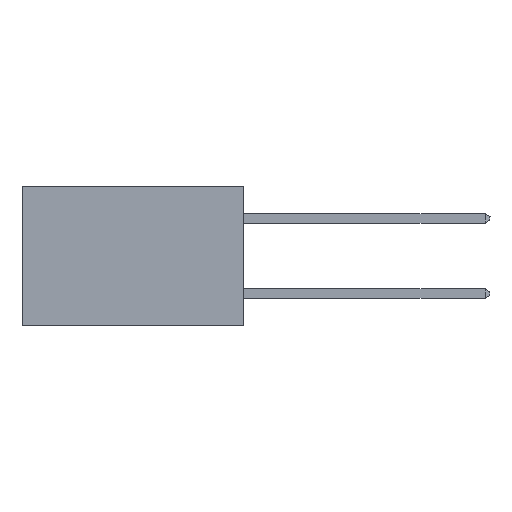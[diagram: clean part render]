
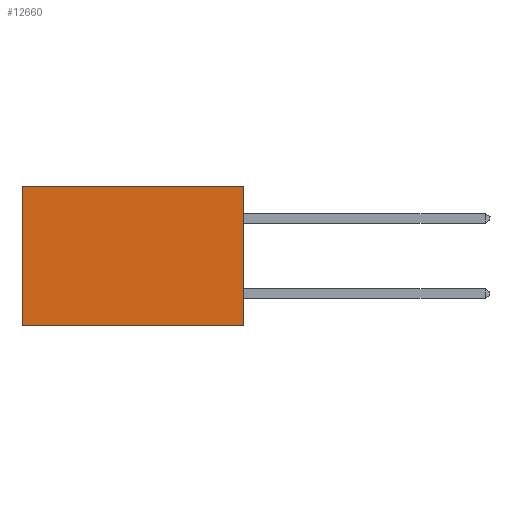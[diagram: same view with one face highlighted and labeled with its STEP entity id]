
A CAD part, left-side view. The second image highlights one B-rep face of the part: STEP entity #12660.
In plain terms, the highlighted planar face has unit normal (-1, 0, 0).
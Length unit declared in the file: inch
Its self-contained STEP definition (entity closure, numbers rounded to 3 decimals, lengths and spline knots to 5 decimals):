
#1228 = DIRECTION ( 'NONE',  ( 0., 0., -1. ) ) ;
#1607 = DIRECTION ( 'NONE',  ( 0., 0., -1. ) ) ;
#2032 = DIRECTION ( 'NONE',  ( 0., 0., -1. ) ) ;
#3193 = EDGE_CURVE ( 'NONE', #11809, #32830, #10603, .T. ) ;
#3891 = ORIENTED_EDGE ( 'NONE', *, *, #25539, .T. ) ;
#6457 = EDGE_LOOP ( 'NONE', ( #3891, #24200, #34186, #10453 ) ) ;
#7240 = LINE ( 'NONE', #34253, #28604 ) ;
#9382 = PLANE ( 'NONE',  #17076 ) ;
#9426 = VECTOR ( 'NONE', #14300, 39.37008 ) ;
#10267 = LINE ( 'NONE', #11620, #9426 ) ;
#10453 = ORIENTED_EDGE ( 'NONE', *, *, #3193, .T. ) ;
#10603 = LINE ( 'NONE', #23053, #30261 ) ;
#11620 = CARTESIAN_POINT ( 'NONE',  ( 0.277, 0., -0.37 ) ) ;
#11809 = VERTEX_POINT ( 'NONE', #30254 ) ;
#12660 = ADVANCED_FACE ( 'NONE', ( #26152 ), #9382, .F. ) ;
#14300 = DIRECTION ( 'NONE',  ( 0., 1., 0. ) ) ;
#15114 = CARTESIAN_POINT ( 'NONE',  ( 0.277, 0.59, -0.37 ) ) ;
#16032 = CARTESIAN_POINT ( 'NONE',  ( 0.277, 0., -0.37 ) ) ;
#17076 = AXIS2_PLACEMENT_3D ( 'NONE', #33505, #17491, #1228 ) ;
#17491 = DIRECTION ( 'NONE',  ( 1., 0., 0. ) ) ;
#19678 = LINE ( 'NONE', #15114, #32180 ) ;
#22779 = CARTESIAN_POINT ( 'NONE',  ( 0.277, 0.59, -0.37 ) ) ;
#23053 = CARTESIAN_POINT ( 'NONE',  ( 0.277, 0., 0. ) ) ;
#24200 = ORIENTED_EDGE ( 'NONE', *, *, #27353, .F. ) ;
#25451 = VERTEX_POINT ( 'NONE', #22779 ) ;
#25539 = EDGE_CURVE ( 'NONE', #32830, #25451, #19678, .T. ) ;
#25706 = CARTESIAN_POINT ( 'NONE',  ( 0.277, 0.59, 0. ) ) ;
#26152 = FACE_OUTER_BOUND ( 'NONE', #6457, .T. ) ;
#27353 = EDGE_CURVE ( 'NONE', #34421, #25451, #10267, .T. ) ;
#28604 = VECTOR ( 'NONE', #2032, 39.37008 ) ;
#28611 = EDGE_CURVE ( 'NONE', #11809, #34421, #7240, .T. ) ;
#30254 = CARTESIAN_POINT ( 'NONE',  ( 0.277, 0., 0. ) ) ;
#30261 = VECTOR ( 'NONE', #32451, 39.37008 ) ;
#32180 = VECTOR ( 'NONE', #1607, 39.37008 ) ;
#32451 = DIRECTION ( 'NONE',  ( 0., 1., 0. ) ) ;
#32830 = VERTEX_POINT ( 'NONE', #25706 ) ;
#33505 = CARTESIAN_POINT ( 'NONE',  ( 0.277, 0., -0.37 ) ) ;
#34186 = ORIENTED_EDGE ( 'NONE', *, *, #28611, .F. ) ;
#34253 = CARTESIAN_POINT ( 'NONE',  ( 0.277, 0., -0.37 ) ) ;
#34421 = VERTEX_POINT ( 'NONE', #16032 ) ;
